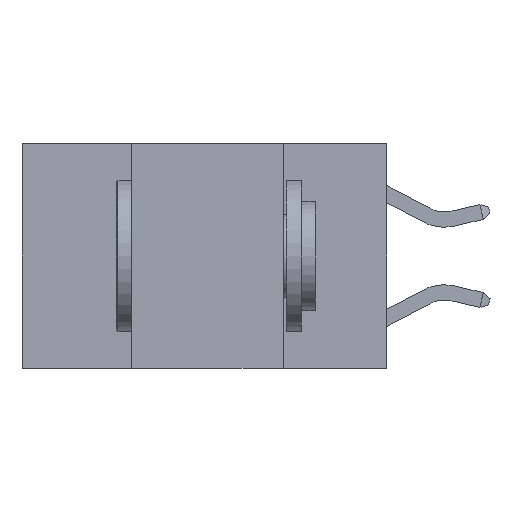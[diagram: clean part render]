
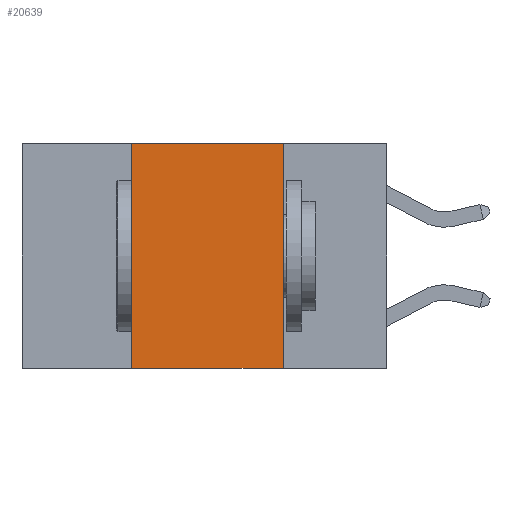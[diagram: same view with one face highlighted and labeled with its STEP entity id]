
A CAD part, left-side view. The second image highlights one B-rep face of the part: STEP entity #20639.
In plain terms, the highlighted planar face has unit normal (-1, 0, 0).
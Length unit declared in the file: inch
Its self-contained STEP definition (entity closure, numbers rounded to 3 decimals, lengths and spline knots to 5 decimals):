
#429 = CARTESIAN_POINT ( 'NONE',  ( 0., 0.6, 0. ) ) ;
#2082 = DIRECTION ( 'NONE',  ( 0., 0., -1. ) ) ;
#2420 = CARTESIAN_POINT ( 'NONE',  ( 0., 0.42, 0. ) ) ;
#4329 = LINE ( 'NONE', #19552, #28089 ) ;
#4508 = DIRECTION ( 'NONE',  ( 0., -1., 0. ) ) ;
#5751 = CARTESIAN_POINT ( 'NONE',  ( 0., 0.6, 0. ) ) ;
#6741 = CARTESIAN_POINT ( 'NONE',  ( 0., 0.17, -0.37 ) ) ;
#7076 = EDGE_LOOP ( 'NONE', ( #18672, #10590, #31020, #25373 ) ) ;
#7777 = EDGE_CURVE ( 'NONE', #14685, #28277, #24986, .T. ) ;
#8199 = EDGE_CURVE ( 'NONE', #14685, #26794, #4329, .T. ) ;
#8401 = LINE ( 'NONE', #5751, #19025 ) ;
#8905 = DIRECTION ( 'NONE',  ( 0., 0., 1. ) ) ;
#10257 = CARTESIAN_POINT ( 'NONE',  ( 0., 0.42, 0. ) ) ;
#10590 = ORIENTED_EDGE ( 'NONE', *, *, #24635, .F. ) ;
#10958 = PLANE ( 'NONE',  #17715 ) ;
#12511 = CARTESIAN_POINT ( 'NONE',  ( 0., 0.42, -0.37 ) ) ;
#14685 = VERTEX_POINT ( 'NONE', #12511 ) ;
#15264 = VECTOR ( 'NONE', #2082, 39.37008 ) ;
#15957 = VECTOR ( 'NONE', #8905, 39.37008 ) ;
#17379 = CARTESIAN_POINT ( 'NONE',  ( 0., 0.17, 0. ) ) ;
#17715 = AXIS2_PLACEMENT_3D ( 'NONE', #429, #20399, #30872 ) ;
#18672 = ORIENTED_EDGE ( 'NONE', *, *, #23487, .F. ) ;
#19025 = VECTOR ( 'NONE', #25715, 39.37008 ) ;
#19338 = LINE ( 'NONE', #24978, #15264 ) ;
#19552 = CARTESIAN_POINT ( 'NONE',  ( 0., 0.6, -0.37 ) ) ;
#20399 = DIRECTION ( 'NONE',  ( 1., 0., 0. ) ) ;
#20639 = ADVANCED_FACE ( 'NONE', ( #22847 ), #10958, .F. ) ;
#22847 = FACE_OUTER_BOUND ( 'NONE', #7076, .T. ) ;
#23487 = EDGE_CURVE ( 'NONE', #23764, #26794, #19338, .T. ) ;
#23764 = VERTEX_POINT ( 'NONE', #17379 ) ;
#24635 = EDGE_CURVE ( 'NONE', #28277, #23764, #8401, .T. ) ;
#24978 = CARTESIAN_POINT ( 'NONE',  ( 0., 0.17, 0. ) ) ;
#24986 = LINE ( 'NONE', #2420, #15957 ) ;
#25373 = ORIENTED_EDGE ( 'NONE', *, *, #8199, .T. ) ;
#25715 = DIRECTION ( 'NONE',  ( 0., -1., 0. ) ) ;
#26794 = VERTEX_POINT ( 'NONE', #6741 ) ;
#28089 = VECTOR ( 'NONE', #4508, 39.37008 ) ;
#28277 = VERTEX_POINT ( 'NONE', #10257 ) ;
#30872 = DIRECTION ( 'NONE',  ( 0., 0., -1. ) ) ;
#31020 = ORIENTED_EDGE ( 'NONE', *, *, #7777, .F. ) ;
